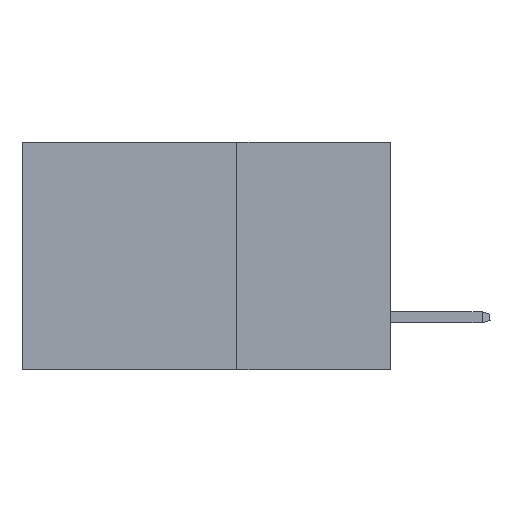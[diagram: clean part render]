
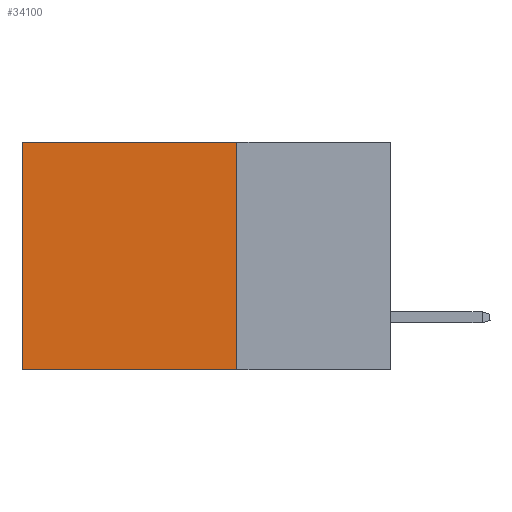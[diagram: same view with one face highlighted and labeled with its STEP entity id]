
A CAD part, left-side view. The second image highlights one B-rep face of the part: STEP entity #34100.
In plain terms, the highlighted planar face has unit normal (-1, 0, 0).
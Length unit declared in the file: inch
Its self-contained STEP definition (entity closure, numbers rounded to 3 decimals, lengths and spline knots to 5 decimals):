
#1915 = CARTESIAN_POINT ( 'NONE',  ( 0.2875, 0.25, 0. ) ) ;
#3551 = VERTEX_POINT ( 'NONE', #14898 ) ;
#4355 = EDGE_CURVE ( 'NONE', #39812, #32756, #43602, .T. ) ;
#5211 = CARTESIAN_POINT ( 'NONE',  ( 0.2875, 0.25, 0. ) ) ;
#6671 = AXIS2_PLACEMENT_3D ( 'NONE', #1915, #48262, #21024 ) ;
#7586 = CARTESIAN_POINT ( 'NONE',  ( 0.2875, 0.25, -0.37 ) ) ;
#8935 = DIRECTION ( 'NONE',  ( 0., 0., -1. ) ) ;
#12635 = ORIENTED_EDGE ( 'NONE', *, *, #23334, .T. ) ;
#12854 = CARTESIAN_POINT ( 'NONE',  ( 0.2875, 0.25, 0. ) ) ;
#12950 = FACE_OUTER_BOUND ( 'NONE', #38821, .T. ) ;
#13921 = ORIENTED_EDGE ( 'NONE', *, *, #4355, .T. ) ;
#14898 = CARTESIAN_POINT ( 'NONE',  ( 0.2875, 0.6, -0.37 ) ) ;
#15431 = VECTOR ( 'NONE', #37188, 39.37008 ) ;
#16359 = EDGE_CURVE ( 'NONE', #39812, #18124, #46836, .T. ) ;
#18124 = VERTEX_POINT ( 'NONE', #7586 ) ;
#18583 = DIRECTION ( 'NONE',  ( 0., 1., 0. ) ) ;
#19764 = EDGE_CURVE ( 'NONE', #18124, #3551, #37262, .T. ) ;
#21024 = DIRECTION ( 'NONE',  ( 0., 0., -1. ) ) ;
#22326 = VECTOR ( 'NONE', #8935, 39.37008 ) ;
#23216 = CARTESIAN_POINT ( 'NONE',  ( 0.2875, 0.25, 0. ) ) ;
#23334 = EDGE_CURVE ( 'NONE', #32756, #3551, #45949, .T. ) ;
#23861 = VECTOR ( 'NONE', #47266, 39.37008 ) ;
#31898 = VECTOR ( 'NONE', #18583, 39.37008 ) ;
#32756 = VERTEX_POINT ( 'NONE', #34165 ) ;
#34100 = ADVANCED_FACE ( 'NONE', ( #12950 ), #36224, .F. ) ;
#34165 = CARTESIAN_POINT ( 'NONE',  ( 0.2875, 0.6, 0. ) ) ;
#36224 = PLANE ( 'NONE',  #6671 ) ;
#37188 = DIRECTION ( 'NONE',  ( 0., 0., -1. ) ) ;
#37262 = LINE ( 'NONE', #40217, #31898 ) ;
#38821 = EDGE_LOOP ( 'NONE', ( #12635, #47260, #47899, #13921 ) ) ;
#39812 = VERTEX_POINT ( 'NONE', #23216 ) ;
#40217 = CARTESIAN_POINT ( 'NONE',  ( 0.2875, 0.25, -0.37 ) ) ;
#43602 = LINE ( 'NONE', #12854, #23861 ) ;
#45949 = LINE ( 'NONE', #48066, #15431 ) ;
#46836 = LINE ( 'NONE', #5211, #22326 ) ;
#47260 = ORIENTED_EDGE ( 'NONE', *, *, #19764, .F. ) ;
#47266 = DIRECTION ( 'NONE',  ( 0., 1., 0. ) ) ;
#47899 = ORIENTED_EDGE ( 'NONE', *, *, #16359, .F. ) ;
#48066 = CARTESIAN_POINT ( 'NONE',  ( 0.2875, 0.6, 0. ) ) ;
#48262 = DIRECTION ( 'NONE',  ( 1., 0., 0. ) ) ;
